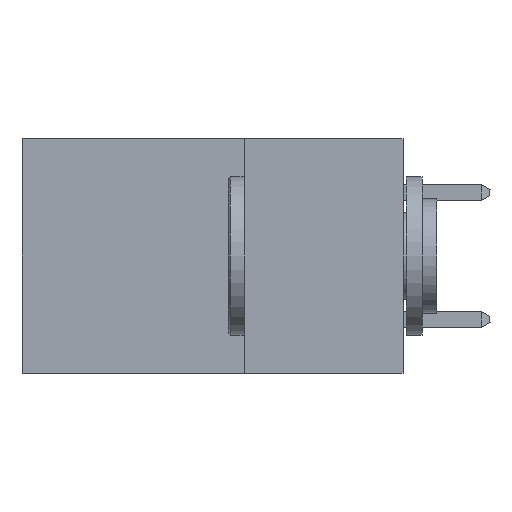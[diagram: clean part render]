
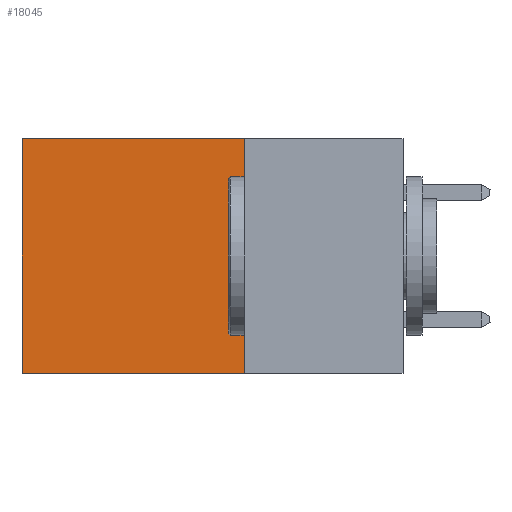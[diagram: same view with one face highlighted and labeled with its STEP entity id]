
A CAD part, left-side view. The second image highlights one B-rep face of the part: STEP entity #18045.
In plain terms, the highlighted planar face has unit normal (-1, 0, 0).
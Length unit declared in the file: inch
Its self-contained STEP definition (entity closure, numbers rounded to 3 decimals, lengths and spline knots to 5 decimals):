
#179 = CARTESIAN_POINT ( 'NONE',  ( 0.2875, 0.25, -0.37 ) ) ;
#700 = AXIS2_PLACEMENT_3D ( 'NONE', #5913, #10275, #1603 ) ;
#1603 = DIRECTION ( 'NONE',  ( 0., 0., -1. ) ) ;
#2234 = CARTESIAN_POINT ( 'NONE',  ( 0.2875, 0.25, 0. ) ) ;
#2795 = VECTOR ( 'NONE', #4489, 39.37008 ) ;
#2802 = DIRECTION ( 'NONE',  ( 0., 0., -1. ) ) ;
#3197 = LINE ( 'NONE', #4291, #14223 ) ;
#3326 = VERTEX_POINT ( 'NONE', #2234 ) ;
#4256 = CARTESIAN_POINT ( 'NONE',  ( 0.2875, 0.25, 0. ) ) ;
#4291 = CARTESIAN_POINT ( 'NONE',  ( 0.2875, 0.25, 0. ) ) ;
#4489 = DIRECTION ( 'NONE',  ( 0., 1., 0. ) ) ;
#5706 = CARTESIAN_POINT ( 'NONE',  ( 0.2875, 0.6, 0. ) ) ;
#5747 = DIRECTION ( 'NONE',  ( 0., 1., 0. ) ) ;
#5798 = VECTOR ( 'NONE', #14873, 39.37008 ) ;
#5913 = CARTESIAN_POINT ( 'NONE',  ( 0.2875, 0.25, 0. ) ) ;
#6335 = ORIENTED_EDGE ( 'NONE', *, *, #11696, .F. ) ;
#6662 = LINE ( 'NONE', #13112, #2795 ) ;
#7327 = ORIENTED_EDGE ( 'NONE', *, *, #14154, .F. ) ;
#7345 = PLANE ( 'NONE',  #700 ) ;
#9270 = FACE_OUTER_BOUND ( 'NONE', #18431, .T. ) ;
#9651 = LINE ( 'NONE', #10553, #5798 ) ;
#10166 = VECTOR ( 'NONE', #2802, 39.37008 ) ;
#10275 = DIRECTION ( 'NONE',  ( 1., 0., 0. ) ) ;
#10553 = CARTESIAN_POINT ( 'NONE',  ( 0.2875, 0.6, 0. ) ) ;
#11696 = EDGE_CURVE ( 'NONE', #12402, #13138, #6662, .T. ) ;
#12402 = VERTEX_POINT ( 'NONE', #179 ) ;
#13112 = CARTESIAN_POINT ( 'NONE',  ( 0.2875, 0.25, -0.37 ) ) ;
#13138 = VERTEX_POINT ( 'NONE', #17955 ) ;
#13484 = EDGE_CURVE ( 'NONE', #3326, #15917, #3197, .T. ) ;
#14115 = ORIENTED_EDGE ( 'NONE', *, *, #16708, .T. ) ;
#14154 = EDGE_CURVE ( 'NONE', #3326, #12402, #17792, .T. ) ;
#14223 = VECTOR ( 'NONE', #5747, 39.37008 ) ;
#14873 = DIRECTION ( 'NONE',  ( 0., 0., -1. ) ) ;
#15917 = VERTEX_POINT ( 'NONE', #5706 ) ;
#16708 = EDGE_CURVE ( 'NONE', #15917, #13138, #9651, .T. ) ;
#16734 = ORIENTED_EDGE ( 'NONE', *, *, #13484, .T. ) ;
#17792 = LINE ( 'NONE', #4256, #10166 ) ;
#17955 = CARTESIAN_POINT ( 'NONE',  ( 0.2875, 0.6, -0.37 ) ) ;
#18045 = ADVANCED_FACE ( 'NONE', ( #9270 ), #7345, .F. ) ;
#18431 = EDGE_LOOP ( 'NONE', ( #14115, #6335, #7327, #16734 ) ) ;
